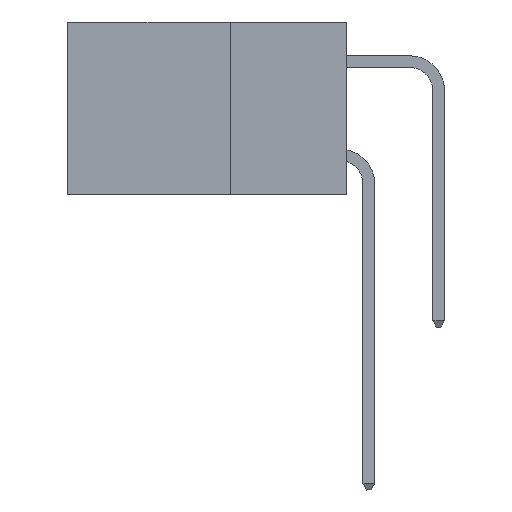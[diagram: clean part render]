
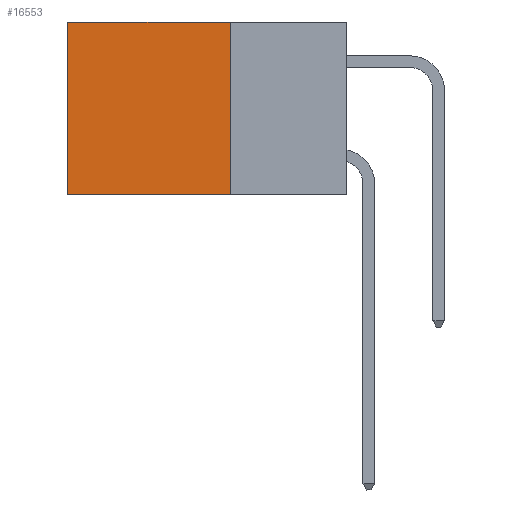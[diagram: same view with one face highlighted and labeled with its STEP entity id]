
A CAD part, left-side view. The second image highlights one B-rep face of the part: STEP entity #16553.
In plain terms, the highlighted planar face has unit normal (-1, 0, 0).
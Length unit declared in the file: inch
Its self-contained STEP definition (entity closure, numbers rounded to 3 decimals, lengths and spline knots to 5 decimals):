
#47 = ORIENTED_EDGE ( 'NONE', *, *, #20935, .T. ) ;
#152 = ORIENTED_EDGE ( 'NONE', *, *, #16348, .T. ) ;
#178 = CARTESIAN_POINT ( 'NONE',  ( 0.2875, 0.25, -0.37 ) ) ;
#340 = VERTEX_POINT ( 'NONE', #7015 ) ;
#526 = EDGE_CURVE ( 'NONE', #2421, #576, #9632, .T. ) ;
#576 = VERTEX_POINT ( 'NONE', #7672 ) ;
#1475 = DIRECTION ( 'NONE',  ( 0., 1., 0. ) ) ;
#2421 = VERTEX_POINT ( 'NONE', #18723 ) ;
#2438 = DIRECTION ( 'NONE',  ( 0., 0., -1. ) ) ;
#7015 = CARTESIAN_POINT ( 'NONE',  ( 0.2875, 0.6, 0. ) ) ;
#7483 = LINE ( 'NONE', #22311, #17410 ) ;
#7522 = DIRECTION ( 'NONE',  ( 0., 1., 0. ) ) ;
#7672 = CARTESIAN_POINT ( 'NONE',  ( 0.2875, 0.6, -0.37 ) ) ;
#9120 = DIRECTION ( 'NONE',  ( 0., 0., -1. ) ) ;
#9204 = VECTOR ( 'NONE', #9120, 39.37008 ) ;
#9632 = LINE ( 'NONE', #178, #18840 ) ;
#10117 = PLANE ( 'NONE',  #18730 ) ;
#10622 = EDGE_LOOP ( 'NONE', ( #152, #15441, #20235, #47 ) ) ;
#11513 = CARTESIAN_POINT ( 'NONE',  ( 0.2875, 0.25, 0. ) ) ;
#12051 = CARTESIAN_POINT ( 'NONE',  ( 0.2875, 0.25, 0. ) ) ;
#12271 = LINE ( 'NONE', #23767, #21326 ) ;
#12272 = FACE_OUTER_BOUND ( 'NONE', #10622, .T. ) ;
#13388 = DIRECTION ( 'NONE',  ( 0., 0., -1. ) ) ;
#13942 = DIRECTION ( 'NONE',  ( 1., 0., 0. ) ) ;
#15441 = ORIENTED_EDGE ( 'NONE', *, *, #526, .F. ) ;
#16348 = EDGE_CURVE ( 'NONE', #340, #576, #7483, .T. ) ;
#16553 = ADVANCED_FACE ( 'NONE', ( #12272 ), #10117, .F. ) ;
#17410 = VECTOR ( 'NONE', #13388, 39.37008 ) ;
#18723 = CARTESIAN_POINT ( 'NONE',  ( 0.2875, 0.25, -0.37 ) ) ;
#18730 = AXIS2_PLACEMENT_3D ( 'NONE', #12051, #13942, #2438 ) ;
#18840 = VECTOR ( 'NONE', #7522, 39.37008 ) ;
#19574 = LINE ( 'NONE', #23711, #9204 ) ;
#19623 = VERTEX_POINT ( 'NONE', #11513 ) ;
#20235 = ORIENTED_EDGE ( 'NONE', *, *, #23283, .F. ) ;
#20935 = EDGE_CURVE ( 'NONE', #19623, #340, #12271, .T. ) ;
#21326 = VECTOR ( 'NONE', #1475, 39.37008 ) ;
#22311 = CARTESIAN_POINT ( 'NONE',  ( 0.2875, 0.6, 0. ) ) ;
#23283 = EDGE_CURVE ( 'NONE', #19623, #2421, #19574, .T. ) ;
#23711 = CARTESIAN_POINT ( 'NONE',  ( 0.2875, 0.25, 0. ) ) ;
#23767 = CARTESIAN_POINT ( 'NONE',  ( 0.2875, 0.25, 0. ) ) ;
